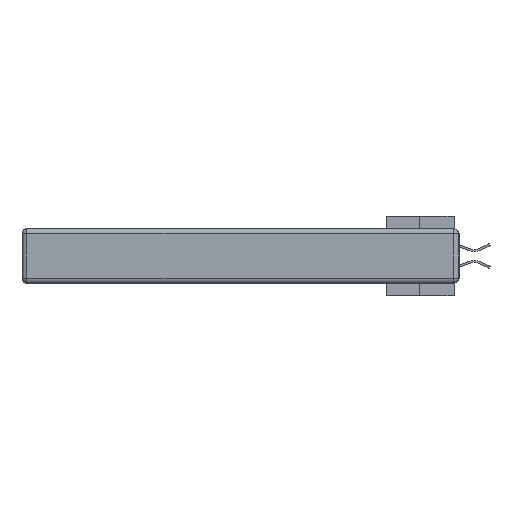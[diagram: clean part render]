
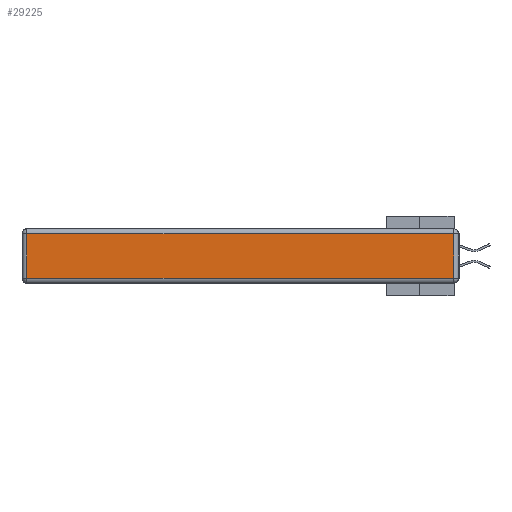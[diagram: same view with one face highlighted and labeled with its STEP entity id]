
A CAD part, left-side view. The second image highlights one B-rep face of the part: STEP entity #29225.
In plain terms, the highlighted planar face has unit normal (-1, 0, 0).
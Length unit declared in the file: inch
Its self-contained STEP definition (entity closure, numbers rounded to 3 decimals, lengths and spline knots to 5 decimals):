
#815 = EDGE_CURVE ( 'NONE', #46633, #19896, #46456, .T. ) ;
#1349 = ORIENTED_EDGE ( 'NONE', *, *, #2679, .T. ) ;
#1362 = LINE ( 'NONE', #22083, #19249 ) ;
#2679 = EDGE_CURVE ( 'NONE', #35388, #46633, #37360, .T. ) ;
#4026 = PLANE ( 'NONE',  #38640 ) ;
#8965 = EDGE_CURVE ( 'NONE', #19896, #8981, #1362, .T. ) ;
#8981 = VERTEX_POINT ( 'NONE', #48442 ) ;
#9839 = DIRECTION ( 'NONE',  ( 0., 0., -1. ) ) ;
#10489 = FACE_OUTER_BOUND ( 'NONE', #15379, .T. ) ;
#14402 = DIRECTION ( 'NONE',  ( 0., 0., 1. ) ) ;
#15379 = EDGE_LOOP ( 'NONE', ( #45877, #38685, #37217, #1349 ) ) ;
#16565 = DIRECTION ( 'NONE',  ( 0., -1., 0. ) ) ;
#17002 = CARTESIAN_POINT ( 'NONE',  ( 0., 2.72, -0.343 ) ) ;
#18731 = DIRECTION ( 'NONE',  ( -1., 0., 0. ) ) ;
#19249 = VECTOR ( 'NONE', #14402, 39.37008 ) ;
#19896 = VERTEX_POINT ( 'NONE', #20492 ) ;
#20226 = CARTESIAN_POINT ( 'NONE',  ( 0., 0., -0.313 ) ) ;
#20492 = CARTESIAN_POINT ( 'NONE',  ( 0., 0.03, -0.313 ) ) ;
#22083 = CARTESIAN_POINT ( 'NONE',  ( 0., 0.03, -0.343 ) ) ;
#24409 = VECTOR ( 'NONE', #16565, 39.37008 ) ;
#29225 = ADVANCED_FACE ( 'NONE', ( #10489 ), #4026, .T. ) ;
#30675 = DIRECTION ( 'NONE',  ( 0., 0., 1. ) ) ;
#33494 = VECTOR ( 'NONE', #33577, 39.37008 ) ;
#33577 = DIRECTION ( 'NONE',  ( 0., 1., 0. ) ) ;
#34084 = CARTESIAN_POINT ( 'NONE',  ( 0., 2.75, -0.03 ) ) ;
#35388 = VERTEX_POINT ( 'NONE', #41421 ) ;
#37217 = ORIENTED_EDGE ( 'NONE', *, *, #47424, .T. ) ;
#37360 = LINE ( 'NONE', #17002, #49288 ) ;
#38640 = AXIS2_PLACEMENT_3D ( 'NONE', #45550, #18731, #30675 ) ;
#38685 = ORIENTED_EDGE ( 'NONE', *, *, #8965, .T. ) ;
#41421 = CARTESIAN_POINT ( 'NONE',  ( 0., 2.72, -0.03 ) ) ;
#43660 = LINE ( 'NONE', #34084, #33494 ) ;
#44380 = CARTESIAN_POINT ( 'NONE',  ( 0., 2.72, -0.313 ) ) ;
#45550 = CARTESIAN_POINT ( 'NONE',  ( 0., 0., -0.343 ) ) ;
#45877 = ORIENTED_EDGE ( 'NONE', *, *, #815, .T. ) ;
#46456 = LINE ( 'NONE', #20226, #24409 ) ;
#46633 = VERTEX_POINT ( 'NONE', #44380 ) ;
#47424 = EDGE_CURVE ( 'NONE', #8981, #35388, #43660, .T. ) ;
#48442 = CARTESIAN_POINT ( 'NONE',  ( 0., 0.03, -0.03 ) ) ;
#49288 = VECTOR ( 'NONE', #9839, 39.37008 ) ;
